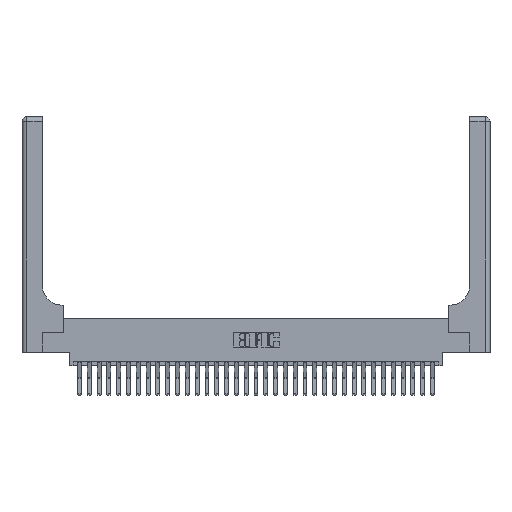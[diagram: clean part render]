
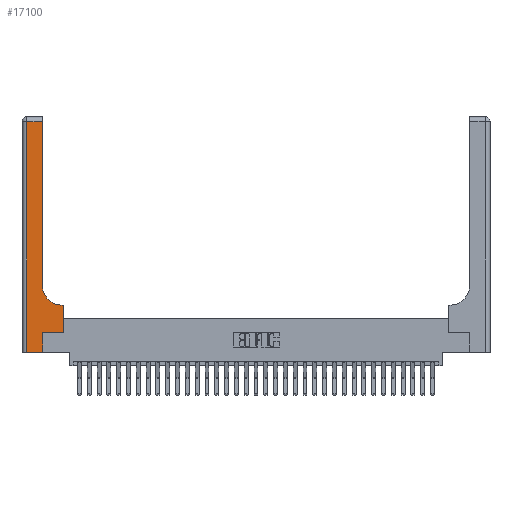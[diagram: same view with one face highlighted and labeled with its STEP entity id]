
A CAD part, top view. The second image highlights one B-rep face of the part: STEP entity #17100.
In plain terms, the highlighted planar face has unit normal (0, 0, 1).
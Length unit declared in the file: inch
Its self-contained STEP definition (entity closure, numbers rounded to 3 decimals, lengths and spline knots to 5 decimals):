
#31 = CARTESIAN_POINT ( 'NONE',  ( 0., 2.94, 0.37 ) ) ;
#143 = VECTOR ( 'NONE', #17642, 39.37008 ) ;
#403 = CARTESIAN_POINT ( 'NONE',  ( 0.528, 0.25, 0.37 ) ) ;
#432 = CARTESIAN_POINT ( 'NONE',  ( 0.528, 0.6, 0.37 ) ) ;
#447 = VECTOR ( 'NONE', #28503, 39.37008 ) ;
#580 = VERTEX_POINT ( 'NONE', #12264 ) ;
#1222 = DIRECTION ( 'NONE',  ( 1., 0., 0. ) ) ;
#1264 = DIRECTION ( 'NONE',  ( 1., 0., 0. ) ) ;
#1286 = LINE ( 'NONE', #26951, #19137 ) ;
#1387 = DIRECTION ( 'NONE',  ( -1., 0., 0. ) ) ;
#1523 = CIRCLE ( 'NONE', #19848, 0.25 ) ;
#1527 = CARTESIAN_POINT ( 'NONE',  ( 0.06, 3., 0.37 ) ) ;
#2322 = ORIENTED_EDGE ( 'NONE', *, *, #25600, .T. ) ;
#3479 = ORIENTED_EDGE ( 'NONE', *, *, #3672, .T. ) ;
#3672 = EDGE_CURVE ( 'NONE', #6684, #19147, #5971, .T. ) ;
#4327 = ORIENTED_EDGE ( 'NONE', *, *, #21255, .T. ) ;
#4369 = LINE ( 'NONE', #24994, #16001 ) ;
#4515 = AXIS2_PLACEMENT_3D ( 'NONE', #29358, #15324, #1387 ) ;
#4708 = VERTEX_POINT ( 'NONE', #9324 ) ;
#5622 = ORIENTED_EDGE ( 'NONE', *, *, #23323, .T. ) ;
#5883 = VECTOR ( 'NONE', #10877, 39.37008 ) ;
#5971 = LINE ( 'NONE', #12135, #447 ) ;
#6182 = VERTEX_POINT ( 'NONE', #17256 ) ;
#6427 = ORIENTED_EDGE ( 'NONE', *, *, #12619, .T. ) ;
#6684 = VERTEX_POINT ( 'NONE', #403 ) ;
#6883 = EDGE_CURVE ( 'NONE', #6182, #6684, #1286, .T. ) ;
#7944 = ORIENTED_EDGE ( 'NONE', *, *, #13797, .T. ) ;
#8663 = CARTESIAN_POINT ( 'NONE',  ( 0.51, 0.6, 0.37 ) ) ;
#9247 = FACE_OUTER_BOUND ( 'NONE', #12899, .T. ) ;
#9324 = CARTESIAN_POINT ( 'NONE',  ( 0.26, 2.94, 0.37 ) ) ;
#9704 = VECTOR ( 'NONE', #19968, 39.37008 ) ;
#10586 = ORIENTED_EDGE ( 'NONE', *, *, #29275, .T. ) ;
#10877 = DIRECTION ( 'NONE',  ( 0., -1., 0. ) ) ;
#11447 = VERTEX_POINT ( 'NONE', #8663 ) ;
#12135 = CARTESIAN_POINT ( 'NONE',  ( 0.528, 0.25, 0.37 ) ) ;
#12264 = CARTESIAN_POINT ( 'NONE',  ( 0.265, 0., 0.37 ) ) ;
#12506 = CARTESIAN_POINT ( 'NONE',  ( 0.265, 0., 0.37 ) ) ;
#12619 = EDGE_CURVE ( 'NONE', #11447, #12636, #1523, .T. ) ;
#12636 = VERTEX_POINT ( 'NONE', #24650 ) ;
#12899 = EDGE_LOOP ( 'NONE', ( #4327, #2322, #28217, #5622, #7944, #29940, #3479, #10586, #6427 ) ) ;
#13797 = EDGE_CURVE ( 'NONE', #580, #6182, #14185, .T. ) ;
#14112 = VERTEX_POINT ( 'NONE', #20587 ) ;
#14185 = LINE ( 'NONE', #12506, #25204 ) ;
#14837 = DIRECTION ( 'NONE',  ( 0., 1., 0. ) ) ;
#15208 = DIRECTION ( 'NONE',  ( 0., 0., -1. ) ) ;
#15324 = DIRECTION ( 'NONE',  ( 0., 0., -1. ) ) ;
#16001 = VECTOR ( 'NONE', #22625, 39.37008 ) ;
#17100 = ADVANCED_FACE ( 'NONE', ( #9247 ), #17587, .F. ) ;
#17256 = CARTESIAN_POINT ( 'NONE',  ( 0.265, 0.25, 0.37 ) ) ;
#17587 = PLANE ( 'NONE',  #4515 ) ;
#17642 = DIRECTION ( 'NONE',  ( 1., 0., 0. ) ) ;
#18690 = DIRECTION ( 'NONE',  ( -1., 0., 0. ) ) ;
#18744 = LINE ( 'NONE', #19977, #143 ) ;
#19137 = VECTOR ( 'NONE', #1222, 39.37008 ) ;
#19147 = VERTEX_POINT ( 'NONE', #432 ) ;
#19848 = AXIS2_PLACEMENT_3D ( 'NONE', #29231, #15208, #1264 ) ;
#19968 = DIRECTION ( 'NONE',  ( 0., 1., 0. ) ) ;
#19977 = CARTESIAN_POINT ( 'NONE',  ( 0., 0., 0.37 ) ) ;
#20587 = CARTESIAN_POINT ( 'NONE',  ( 0.06, 0., 0.37 ) ) ;
#21255 = EDGE_CURVE ( 'NONE', #12636, #4708, #28365, .T. ) ;
#21612 = VERTEX_POINT ( 'NONE', #28158 ) ;
#22059 = VECTOR ( 'NONE', #18690, 39.37008 ) ;
#22349 = CARTESIAN_POINT ( 'NONE',  ( 0.26, 3., 0.37 ) ) ;
#22625 = DIRECTION ( 'NONE',  ( -1., 0., 0. ) ) ;
#23323 = EDGE_CURVE ( 'NONE', #14112, #580, #18744, .T. ) ;
#24278 = LINE ( 'NONE', #31, #22059 ) ;
#24491 = LINE ( 'NONE', #1527, #5883 ) ;
#24650 = CARTESIAN_POINT ( 'NONE',  ( 0.26, 0.85, 0.37 ) ) ;
#24994 = CARTESIAN_POINT ( 'NONE',  ( 0.26, 0.6, 0.37 ) ) ;
#25204 = VECTOR ( 'NONE', #14837, 39.37008 ) ;
#25600 = EDGE_CURVE ( 'NONE', #4708, #21612, #24278, .T. ) ;
#26951 = CARTESIAN_POINT ( 'NONE',  ( 0.265, 0.25, 0.37 ) ) ;
#28158 = CARTESIAN_POINT ( 'NONE',  ( 0.06, 2.94, 0.37 ) ) ;
#28217 = ORIENTED_EDGE ( 'NONE', *, *, #28757, .T. ) ;
#28365 = LINE ( 'NONE', #22349, #9704 ) ;
#28503 = DIRECTION ( 'NONE',  ( 0., 1., 0. ) ) ;
#28757 = EDGE_CURVE ( 'NONE', #21612, #14112, #24491, .T. ) ;
#29231 = CARTESIAN_POINT ( 'NONE',  ( 0.51, 0.85, 0.37 ) ) ;
#29275 = EDGE_CURVE ( 'NONE', #19147, #11447, #4369, .T. ) ;
#29358 = CARTESIAN_POINT ( 'NONE',  ( 0., 3., 0.37 ) ) ;
#29940 = ORIENTED_EDGE ( 'NONE', *, *, #6883, .T. ) ;
